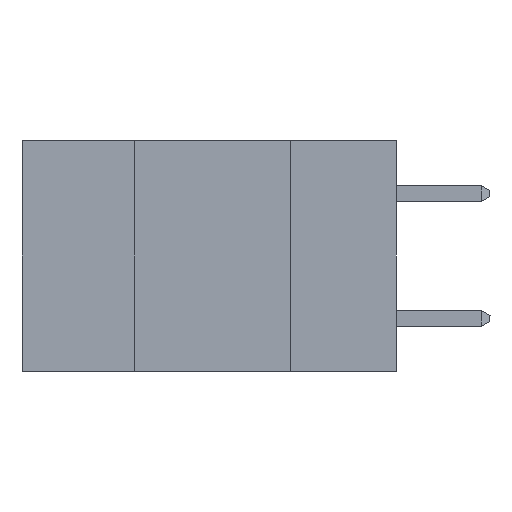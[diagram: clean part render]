
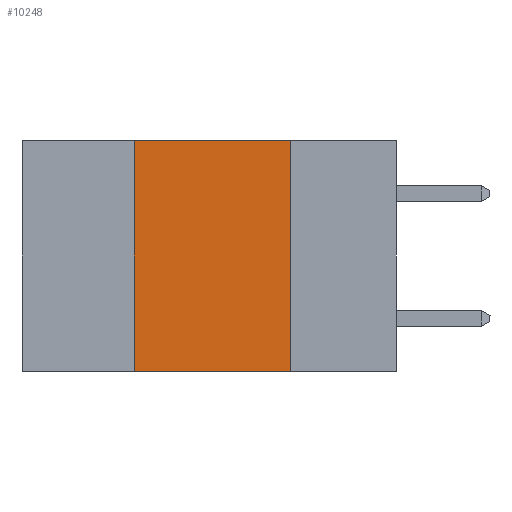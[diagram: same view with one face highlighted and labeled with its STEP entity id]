
A CAD part, left-side view. The second image highlights one B-rep face of the part: STEP entity #10248.
In plain terms, the highlighted planar face has unit normal (-1, 0, 0).
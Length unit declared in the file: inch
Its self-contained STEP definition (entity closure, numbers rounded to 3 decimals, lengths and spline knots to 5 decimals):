
#452 = CARTESIAN_POINT ( 'NONE',  ( 0., 0.6, 0. ) ) ;
#565 = CARTESIAN_POINT ( 'NONE',  ( 0., 0.17, -0.37 ) ) ;
#1211 = VECTOR ( 'NONE', #7344, 39.37008 ) ;
#1820 = DIRECTION ( 'NONE',  ( 0., -1., 0. ) ) ;
#1852 = DIRECTION ( 'NONE',  ( 0., 0., -1. ) ) ;
#1908 = VERTEX_POINT ( 'NONE', #14156 ) ;
#2535 = VECTOR ( 'NONE', #1820, 39.37008 ) ;
#2926 = EDGE_LOOP ( 'NONE', ( #5583, #5638, #5657, #5716 ) ) ;
#3341 = VECTOR ( 'NONE', #11953, 39.37008 ) ;
#3451 = VERTEX_POINT ( 'NONE', #4118 ) ;
#3467 = DIRECTION ( 'NONE',  ( 0., 0., 1. ) ) ;
#4118 = CARTESIAN_POINT ( 'NONE',  ( 0., 0.17, -0.37 ) ) ;
#4534 = CARTESIAN_POINT ( 'NONE',  ( 0., 0.6, 0. ) ) ;
#5017 = AXIS2_PLACEMENT_3D ( 'NONE', #452, #9912, #1852 ) ;
#5583 = ORIENTED_EDGE ( 'NONE', *, *, #16901, .F. ) ;
#5638 = ORIENTED_EDGE ( 'NONE', *, *, #15612, .F. ) ;
#5657 = ORIENTED_EDGE ( 'NONE', *, *, #12632, .F. ) ;
#5716 = ORIENTED_EDGE ( 'NONE', *, *, #10558, .T. ) ;
#6068 = VERTEX_POINT ( 'NONE', #15916 ) ;
#7344 = DIRECTION ( 'NONE',  ( 0., 0., -1. ) ) ;
#7388 = CARTESIAN_POINT ( 'NONE',  ( 0., 0.42, -0.37 ) ) ;
#8570 = PLANE ( 'NONE',  #5017 ) ;
#9624 = VECTOR ( 'NONE', #3467, 39.37008 ) ;
#9912 = DIRECTION ( 'NONE',  ( 1., 0., 0. ) ) ;
#10248 = ADVANCED_FACE ( 'NONE', ( #11989 ), #8570, .F. ) ;
#10516 = LINE ( 'NONE', #10607, #3341 ) ;
#10558 = EDGE_CURVE ( 'NONE', #11963, #3451, #10516, .T. ) ;
#10607 = CARTESIAN_POINT ( 'NONE',  ( 0., 0.6, -0.37 ) ) ;
#11953 = DIRECTION ( 'NONE',  ( 0., -1., 0. ) ) ;
#11963 = VERTEX_POINT ( 'NONE', #15576 ) ;
#11989 = FACE_OUTER_BOUND ( 'NONE', #2926, .T. ) ;
#12632 = EDGE_CURVE ( 'NONE', #11963, #6068, #16333, .T. ) ;
#13584 = LINE ( 'NONE', #4534, #2535 ) ;
#14156 = CARTESIAN_POINT ( 'NONE',  ( 0., 0.17, 0. ) ) ;
#15253 = LINE ( 'NONE', #565, #1211 ) ;
#15576 = CARTESIAN_POINT ( 'NONE',  ( 0., 0.42, -0.37 ) ) ;
#15612 = EDGE_CURVE ( 'NONE', #6068, #1908, #13584, .T. ) ;
#15916 = CARTESIAN_POINT ( 'NONE',  ( 0., 0.42, 0. ) ) ;
#16333 = LINE ( 'NONE', #7388, #9624 ) ;
#16901 = EDGE_CURVE ( 'NONE', #1908, #3451, #15253, .T. ) ;
